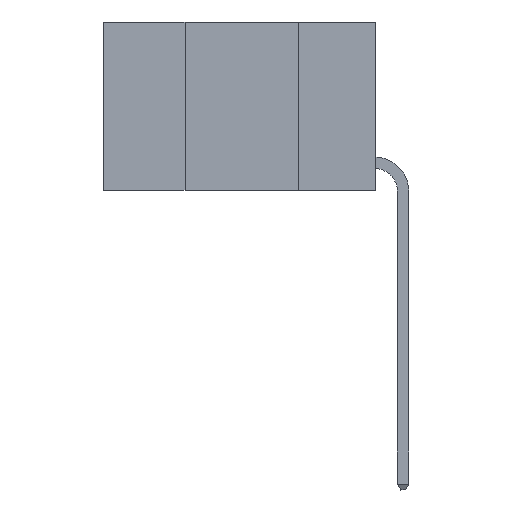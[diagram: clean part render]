
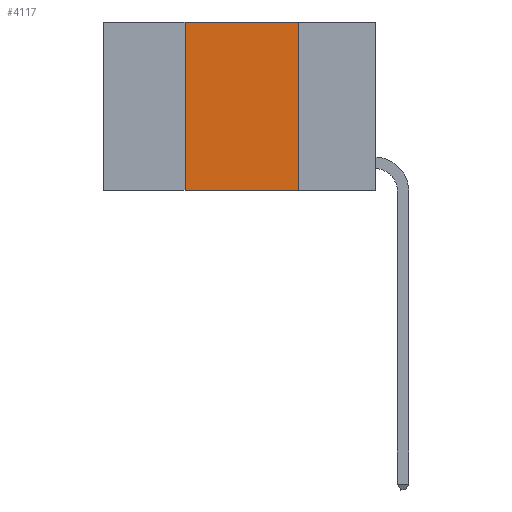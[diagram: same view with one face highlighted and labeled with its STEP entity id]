
A CAD part, left-side view. The second image highlights one B-rep face of the part: STEP entity #4117.
In plain terms, the highlighted planar face has unit normal (-1, 0, 0).
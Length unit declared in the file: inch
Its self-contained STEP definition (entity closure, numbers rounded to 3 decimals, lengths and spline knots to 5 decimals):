
#153 = LINE ( 'NONE', #6510, #16153 ) ;
#320 = CARTESIAN_POINT ( 'NONE',  ( 0., 0.17, -0.37 ) ) ;
#954 = ORIENTED_EDGE ( 'NONE', *, *, #13894, .T. ) ;
#1949 = VERTEX_POINT ( 'NONE', #6106 ) ;
#2641 = EDGE_CURVE ( 'NONE', #13995, #1949, #153, .T. ) ;
#3413 = DIRECTION ( 'NONE',  ( 0., 0., -1. ) ) ;
#3814 = VERTEX_POINT ( 'NONE', #320 ) ;
#4117 = ADVANCED_FACE ( 'NONE', ( #7444 ), #7705, .F. ) ;
#4164 = ORIENTED_EDGE ( 'NONE', *, *, #13694, .F. ) ;
#4407 = CARTESIAN_POINT ( 'NONE',  ( 0., 0.6, -0.37 ) ) ;
#4495 = DIRECTION ( 'NONE',  ( 0., -1., 0. ) ) ;
#4679 = DIRECTION ( 'NONE',  ( 1., 0., 0. ) ) ;
#4700 = EDGE_LOOP ( 'NONE', ( #4164, #6235, #13219, #954 ) ) ;
#4932 = CARTESIAN_POINT ( 'NONE',  ( 0., 0.6, 0. ) ) ;
#5710 = DIRECTION ( 'NONE',  ( 0., -1., 0. ) ) ;
#5802 = LINE ( 'NONE', #4407, #16044 ) ;
#6106 = CARTESIAN_POINT ( 'NONE',  ( 0., 0.42, 0. ) ) ;
#6235 = ORIENTED_EDGE ( 'NONE', *, *, #12806, .F. ) ;
#6446 = VECTOR ( 'NONE', #3413, 39.37008 ) ;
#6510 = CARTESIAN_POINT ( 'NONE',  ( 0., 0.42, 0. ) ) ;
#7258 = LINE ( 'NONE', #12561, #11883 ) ;
#7444 = FACE_OUTER_BOUND ( 'NONE', #4700, .T. ) ;
#7545 = CARTESIAN_POINT ( 'NONE',  ( 0., 0.17, 0. ) ) ;
#7705 = PLANE ( 'NONE',  #14932 ) ;
#9919 = DIRECTION ( 'NONE',  ( 0., 0., -1. ) ) ;
#10948 = DIRECTION ( 'NONE',  ( 0., 0., 1. ) ) ;
#11208 = LINE ( 'NONE', #15374, #6446 ) ;
#11883 = VECTOR ( 'NONE', #4495, 39.37008 ) ;
#12049 = VERTEX_POINT ( 'NONE', #7545 ) ;
#12561 = CARTESIAN_POINT ( 'NONE',  ( 0., 0.6, 0. ) ) ;
#12806 = EDGE_CURVE ( 'NONE', #1949, #12049, #7258, .T. ) ;
#13219 = ORIENTED_EDGE ( 'NONE', *, *, #2641, .F. ) ;
#13431 = CARTESIAN_POINT ( 'NONE',  ( 0., 0.42, -0.37 ) ) ;
#13694 = EDGE_CURVE ( 'NONE', #12049, #3814, #11208, .T. ) ;
#13894 = EDGE_CURVE ( 'NONE', #13995, #3814, #5802, .T. ) ;
#13995 = VERTEX_POINT ( 'NONE', #13431 ) ;
#14932 = AXIS2_PLACEMENT_3D ( 'NONE', #4932, #4679, #9919 ) ;
#15374 = CARTESIAN_POINT ( 'NONE',  ( 0., 0.17, 0. ) ) ;
#16044 = VECTOR ( 'NONE', #5710, 39.37008 ) ;
#16153 = VECTOR ( 'NONE', #10948, 39.37008 ) ;
